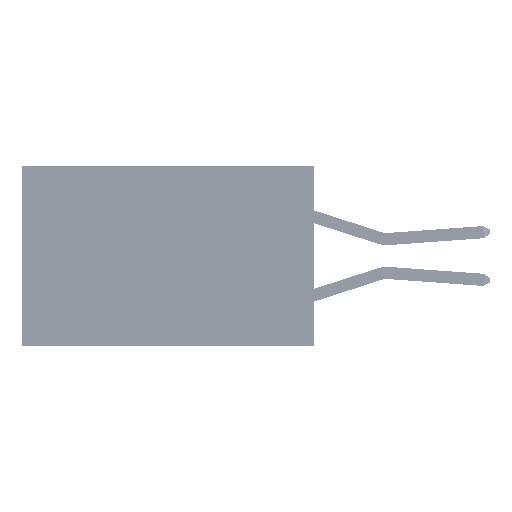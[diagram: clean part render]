
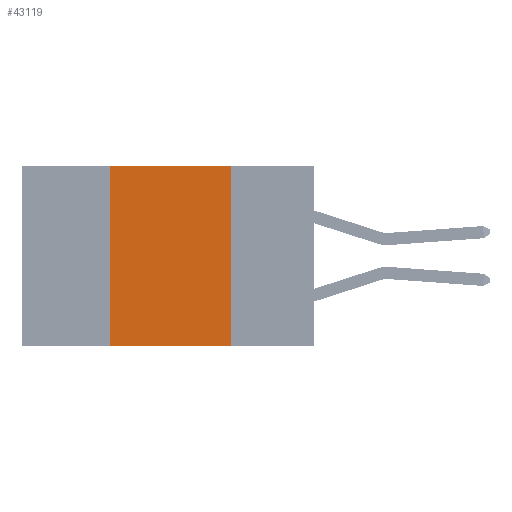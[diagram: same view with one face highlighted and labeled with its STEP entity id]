
A CAD part, left-side view. The second image highlights one B-rep face of the part: STEP entity #43119.
In plain terms, the highlighted planar face has unit normal (-1, 0, 0).
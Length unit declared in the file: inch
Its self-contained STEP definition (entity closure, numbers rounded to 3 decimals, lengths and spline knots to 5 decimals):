
#1709 = VECTOR ( 'NONE', #34628, 39.37008 ) ;
#2578 = DIRECTION ( 'NONE',  ( 0., -1., 0. ) ) ;
#5568 = VERTEX_POINT ( 'NONE', #38914 ) ;
#5845 = VECTOR ( 'NONE', #38328, 39.37008 ) ;
#6566 = LINE ( 'NONE', #43423, #9248 ) ;
#7860 = VECTOR ( 'NONE', #2578, 39.37008 ) ;
#9248 = VECTOR ( 'NONE', #25536, 39.37008 ) ;
#9269 = CARTESIAN_POINT ( 'NONE',  ( 0., 0.42, 0. ) ) ;
#10815 = EDGE_LOOP ( 'NONE', ( #33408, #35216, #16705, #15742 ) ) ;
#11077 = PLANE ( 'NONE',  #25036 ) ;
#13279 = CARTESIAN_POINT ( 'NONE',  ( 0., 0.17, 0. ) ) ;
#13601 = EDGE_CURVE ( 'NONE', #5568, #41025, #18411, .T. ) ;
#14665 = DIRECTION ( 'NONE',  ( 0., 0., -1. ) ) ;
#15742 = ORIENTED_EDGE ( 'NONE', *, *, #26242, .T. ) ;
#16267 = EDGE_CURVE ( 'NONE', #31284, #35422, #19804, .T. ) ;
#16705 = ORIENTED_EDGE ( 'NONE', *, *, #13601, .F. ) ;
#18411 = LINE ( 'NONE', #9269, #1709 ) ;
#19411 = CARTESIAN_POINT ( 'NONE',  ( 0., 0.17, 0. ) ) ;
#19804 = LINE ( 'NONE', #13279, #5845 ) ;
#21690 = DIRECTION ( 'NONE',  ( 1., 0., 0. ) ) ;
#25036 = AXIS2_PLACEMENT_3D ( 'NONE', #42849, #21690, #14665 ) ;
#25536 = DIRECTION ( 'NONE',  ( 0., -1., 0. ) ) ;
#26242 = EDGE_CURVE ( 'NONE', #5568, #35422, #41259, .T. ) ;
#28569 = EDGE_CURVE ( 'NONE', #41025, #31284, #6566, .T. ) ;
#29180 = CARTESIAN_POINT ( 'NONE',  ( 0., 0.42, 0. ) ) ;
#31284 = VERTEX_POINT ( 'NONE', #19411 ) ;
#32286 = FACE_OUTER_BOUND ( 'NONE', #10815, .T. ) ;
#33408 = ORIENTED_EDGE ( 'NONE', *, *, #16267, .F. ) ;
#34628 = DIRECTION ( 'NONE',  ( 0., 0., 1. ) ) ;
#35216 = ORIENTED_EDGE ( 'NONE', *, *, #28569, .F. ) ;
#35422 = VERTEX_POINT ( 'NONE', #40749 ) ;
#38328 = DIRECTION ( 'NONE',  ( 0., 0., -1. ) ) ;
#38914 = CARTESIAN_POINT ( 'NONE',  ( 0., 0.42, -0.37 ) ) ;
#40749 = CARTESIAN_POINT ( 'NONE',  ( 0., 0.17, -0.37 ) ) ;
#41025 = VERTEX_POINT ( 'NONE', #29180 ) ;
#41259 = LINE ( 'NONE', #45369, #7860 ) ;
#42849 = CARTESIAN_POINT ( 'NONE',  ( 0., 0.6, 0. ) ) ;
#43119 = ADVANCED_FACE ( 'NONE', ( #32286 ), #11077, .F. ) ;
#43423 = CARTESIAN_POINT ( 'NONE',  ( 0., 0.6, 0. ) ) ;
#45369 = CARTESIAN_POINT ( 'NONE',  ( 0., 0.6, -0.37 ) ) ;
